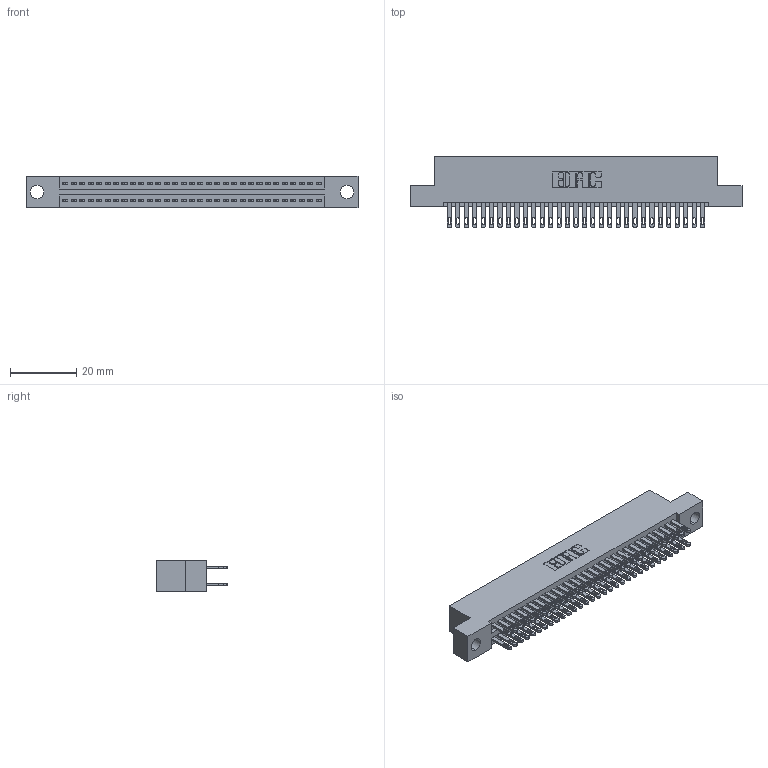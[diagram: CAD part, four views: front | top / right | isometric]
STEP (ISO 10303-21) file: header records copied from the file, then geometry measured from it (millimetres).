
FILE_DESCRIPTION (( 'STEP AP203' ), '1' );
FILE_NAME ('345-062-500-204.STEP', '2021-05-20T05:53:58', ( '' ), ( '' ), 'SwSTEP 2.0', 'SolidWorks 2020', '' );
FILE_SCHEMA (( 'CONFIG_CONTROL_DESIGN' ));
Length unit declared in the file: inch
Products named in the file (3): 345-292-001_345-293-100; 345-062-500-204; 345 Part_Flush Mounting Lugs - 0.156 Dia-TI
Assembly tree (63 placements, depth 2):
  345-062-500-204
    345 Part_Flush Mounting Lugs - 0.156 Dia-TI
    345-292-001_345-293-100  x62
Bounding box: 99.95 x 21.51 x 9.4 mm (x, y, z)
Volume: 9690.6 mm3; surface area: 14595.2 mm2
Topology: 63 solids, 63 shells, 2992 faces, 9119 edges, 6078 vertices
Faces by surface type: plane 1768, cylinder 1224
Entity records: 26153 total; most frequent: CARTESIAN_POINT 4398, ORIENTED_EDGE 4330, DIRECTION 3893, EDGE_CURVE 2165, VECTOR 1905, LINE 1905, VERTEX_POINT 1442, AXIS2_PLACEMENT_3D 994
